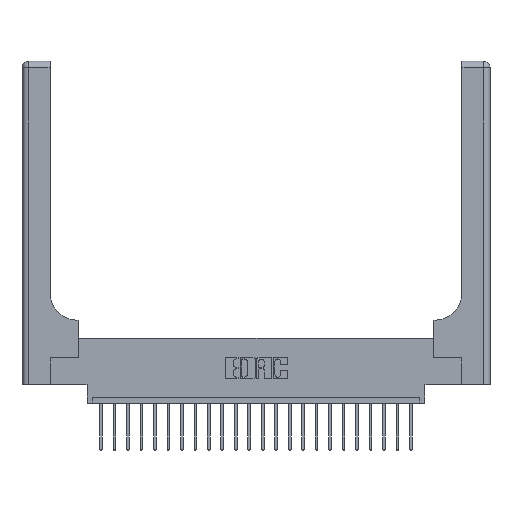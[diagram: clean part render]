
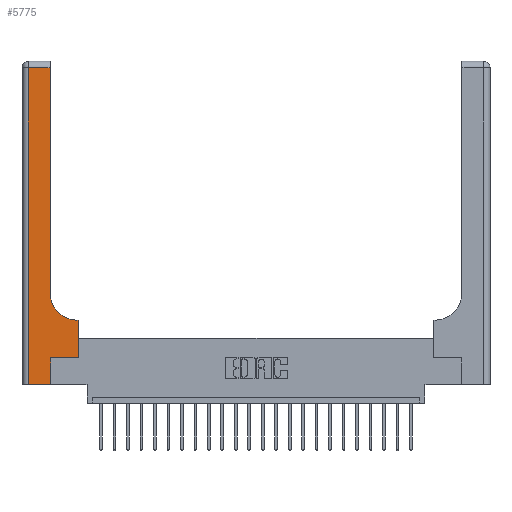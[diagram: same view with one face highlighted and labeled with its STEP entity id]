
A CAD part, top view. The second image highlights one B-rep face of the part: STEP entity #5775.
In plain terms, the highlighted planar face has unit normal (0, 0, 1).
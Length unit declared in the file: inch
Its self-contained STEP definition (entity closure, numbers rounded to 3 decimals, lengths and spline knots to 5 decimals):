
#432 = DIRECTION ( 'NONE',  ( 1., 0., 0. ) ) ;
#826 = PLANE ( 'NONE',  #2268 ) ;
#854 = EDGE_CURVE ( 'NONE', #3191, #6287, #5111, .T. ) ;
#1543 = LINE ( 'NONE', #8695, #18149 ) ;
#1607 = CARTESIAN_POINT ( 'NONE',  ( 0.265, 0.25, 0.37 ) ) ;
#2049 = ORIENTED_EDGE ( 'NONE', *, *, #2907, .T. ) ;
#2074 = VERTEX_POINT ( 'NONE', #2811 ) ;
#2197 = LINE ( 'NONE', #6171, #5838 ) ;
#2268 = AXIS2_PLACEMENT_3D ( 'NONE', #13210, #10925, #11588 ) ;
#2457 = VECTOR ( 'NONE', #15592, 39.37008 ) ;
#2497 = DIRECTION ( 'NONE',  ( 0., 1., 0. ) ) ;
#2587 = ORIENTED_EDGE ( 'NONE', *, *, #21062, .T. ) ;
#2811 = CARTESIAN_POINT ( 'NONE',  ( 0.06, 0., 0.37 ) ) ;
#2907 = EDGE_CURVE ( 'NONE', #6287, #12737, #11393, .T. ) ;
#2976 = LINE ( 'NONE', #10130, #2457 ) ;
#3138 = DIRECTION ( 'NONE',  ( 0., -1., 0. ) ) ;
#3191 = VERTEX_POINT ( 'NONE', #12882 ) ;
#3252 = EDGE_CURVE ( 'NONE', #14810, #3517, #14131, .T. ) ;
#3422 = VECTOR ( 'NONE', #15634, 39.37008 ) ;
#3517 = VERTEX_POINT ( 'NONE', #14253 ) ;
#4000 = DIRECTION ( 'NONE',  ( 0., 0., -1. ) ) ;
#4323 = CARTESIAN_POINT ( 'NONE',  ( 0.528, 0.6, 0.37 ) ) ;
#4603 = ORIENTED_EDGE ( 'NONE', *, *, #19472, .T. ) ;
#4676 = VECTOR ( 'NONE', #16107, 39.37008 ) ;
#5111 = LINE ( 'NONE', #1607, #3422 ) ;
#5775 = ADVANCED_FACE ( 'NONE', ( #17573 ), #826, .F. ) ;
#5838 = VECTOR ( 'NONE', #7464, 39.37008 ) ;
#6171 = CARTESIAN_POINT ( 'NONE',  ( 0.26, 0.6, 0.37 ) ) ;
#6287 = VERTEX_POINT ( 'NONE', #9819 ) ;
#6972 = CARTESIAN_POINT ( 'NONE',  ( 0.26, 2.94, 0.37 ) ) ;
#7464 = DIRECTION ( 'NONE',  ( -1., 0., 0. ) ) ;
#7507 = VERTEX_POINT ( 'NONE', #21640 ) ;
#8419 = LINE ( 'NONE', #10394, #21969 ) ;
#8695 = CARTESIAN_POINT ( 'NONE',  ( 0., 2.94, 0.37 ) ) ;
#8880 = LINE ( 'NONE', #10633, #4676 ) ;
#9036 = CARTESIAN_POINT ( 'NONE',  ( 0.06, 2.94, 0.37 ) ) ;
#9819 = CARTESIAN_POINT ( 'NONE',  ( 0.528, 0.25, 0.37 ) ) ;
#10046 = VERTEX_POINT ( 'NONE', #6972 ) ;
#10130 = CARTESIAN_POINT ( 'NONE',  ( 0.26, 3., 0.37 ) ) ;
#10394 = CARTESIAN_POINT ( 'NONE',  ( 0.06, 3., 0.37 ) ) ;
#10562 = ORIENTED_EDGE ( 'NONE', *, *, #13832, .T. ) ;
#10633 = CARTESIAN_POINT ( 'NONE',  ( 0.265, 0., 0.37 ) ) ;
#10798 = ORIENTED_EDGE ( 'NONE', *, *, #22177, .T. ) ;
#10925 = DIRECTION ( 'NONE',  ( 0., 0., -1. ) ) ;
#10943 = VERTEX_POINT ( 'NONE', #9036 ) ;
#11075 = LINE ( 'NONE', #19704, #15969 ) ;
#11393 = LINE ( 'NONE', #18497, #20112 ) ;
#11588 = DIRECTION ( 'NONE',  ( -1., 0., 0. ) ) ;
#12516 = ORIENTED_EDGE ( 'NONE', *, *, #18060, .T. ) ;
#12737 = VERTEX_POINT ( 'NONE', #4323 ) ;
#12740 = ORIENTED_EDGE ( 'NONE', *, *, #15629, .T. ) ;
#12882 = CARTESIAN_POINT ( 'NONE',  ( 0.265, 0.25, 0.37 ) ) ;
#13210 = CARTESIAN_POINT ( 'NONE',  ( 0., 3., 0.37 ) ) ;
#13832 = EDGE_CURVE ( 'NONE', #3517, #10046, #2976, .T. ) ;
#14131 = CIRCLE ( 'NONE', #18594, 0.25 ) ;
#14253 = CARTESIAN_POINT ( 'NONE',  ( 0.26, 0.85, 0.37 ) ) ;
#14810 = VERTEX_POINT ( 'NONE', #21914 ) ;
#15592 = DIRECTION ( 'NONE',  ( 0., 1., 0. ) ) ;
#15629 = EDGE_CURVE ( 'NONE', #10046, #10943, #1543, .T. ) ;
#15634 = DIRECTION ( 'NONE',  ( 1., 0., 0. ) ) ;
#15969 = VECTOR ( 'NONE', #432, 39.37008 ) ;
#16107 = DIRECTION ( 'NONE',  ( 0., 1., 0. ) ) ;
#16690 = ORIENTED_EDGE ( 'NONE', *, *, #3252, .T. ) ;
#16841 = CARTESIAN_POINT ( 'NONE',  ( 0.51, 0.85, 0.37 ) ) ;
#17573 = FACE_OUTER_BOUND ( 'NONE', #18423, .T. ) ;
#18060 = EDGE_CURVE ( 'NONE', #7507, #3191, #8880, .T. ) ;
#18149 = VECTOR ( 'NONE', #22913, 39.37008 ) ;
#18423 = EDGE_LOOP ( 'NONE', ( #10562, #12740, #10798, #2587, #12516, #19789, #2049, #4603, #16690 ) ) ;
#18497 = CARTESIAN_POINT ( 'NONE',  ( 0.528, 0.25, 0.37 ) ) ;
#18594 = AXIS2_PLACEMENT_3D ( 'NONE', #16841, #4000, #20468 ) ;
#19472 = EDGE_CURVE ( 'NONE', #12737, #14810, #2197, .T. ) ;
#19704 = CARTESIAN_POINT ( 'NONE',  ( 0., 0., 0.37 ) ) ;
#19789 = ORIENTED_EDGE ( 'NONE', *, *, #854, .T. ) ;
#20112 = VECTOR ( 'NONE', #2497, 39.37008 ) ;
#20468 = DIRECTION ( 'NONE',  ( 1., 0., 0. ) ) ;
#21062 = EDGE_CURVE ( 'NONE', #2074, #7507, #11075, .T. ) ;
#21640 = CARTESIAN_POINT ( 'NONE',  ( 0.265, 0., 0.37 ) ) ;
#21914 = CARTESIAN_POINT ( 'NONE',  ( 0.51, 0.6, 0.37 ) ) ;
#21969 = VECTOR ( 'NONE', #3138, 39.37008 ) ;
#22177 = EDGE_CURVE ( 'NONE', #10943, #2074, #8419, .T. ) ;
#22913 = DIRECTION ( 'NONE',  ( -1., 0., 0. ) ) ;
